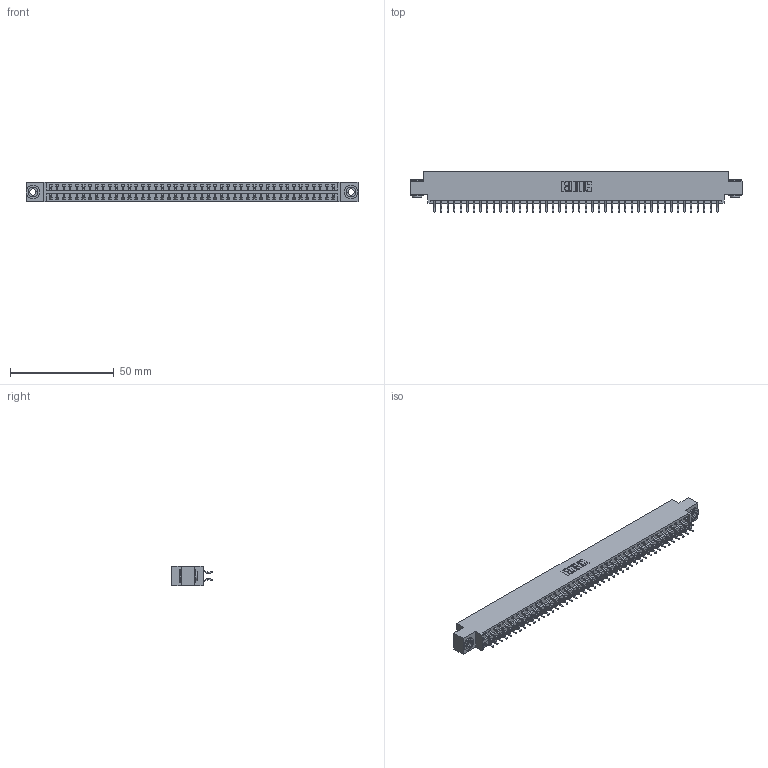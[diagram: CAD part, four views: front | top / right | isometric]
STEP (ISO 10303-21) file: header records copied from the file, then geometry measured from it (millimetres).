
FILE_DESCRIPTION (( 'STEP AP203' ), '1' );
FILE_NAME ('396-088-556-803.STEP', '2018-09-10T06:41:51', ( '' ), ( '' ), 'SwSTEP 2.0', 'SolidWorks 2016', '' );
FILE_SCHEMA (( 'CONFIG_CONTROL_DESIGN' ));
Length unit declared in the file: inch
Products named in the file (4): 396-088-556-803; 346 Part_0.170 Offset - 0.156 Dia-TH; 345-292-001_556 Tail; 345-250-002_345-250-002-102
Assembly tree (91 placements, depth 2):
  396-088-556-803
    346 Part_0.170 Offset - 0.156 Dia-TH
    345-292-001_556 Tail  x88
    345-250-002_345-250-002-102  x2
Bounding box: 160.27 x 19.57 x 9.4 mm (x, y, z)
Volume: 15505.5 mm3; surface area: 21656.9 mm2
Topology: 91 solids, 91 shells, 5268 faces, 15641 edges, 10306 vertices
Faces by surface type: plane 3522, cylinder 1738, cone 8
Entity records: 29448 total; most frequent: CARTESIAN_POINT 4843, ORIENTED_EDGE 4758, DIRECTION 4337, EDGE_CURVE 2379, VECTOR 2039, LINE 2039, VERTEX_POINT 1582, AXIS2_PLACEMENT_3D 1149
